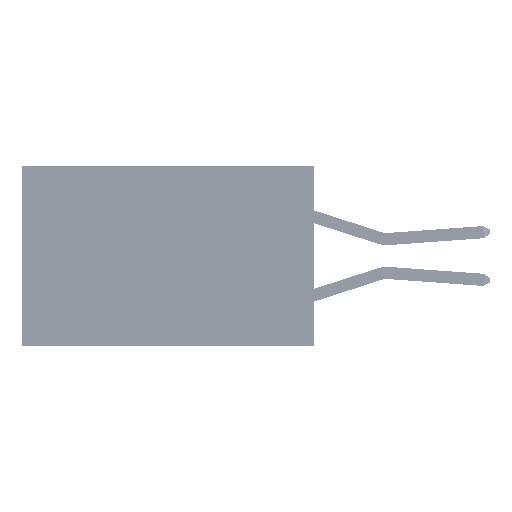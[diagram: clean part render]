
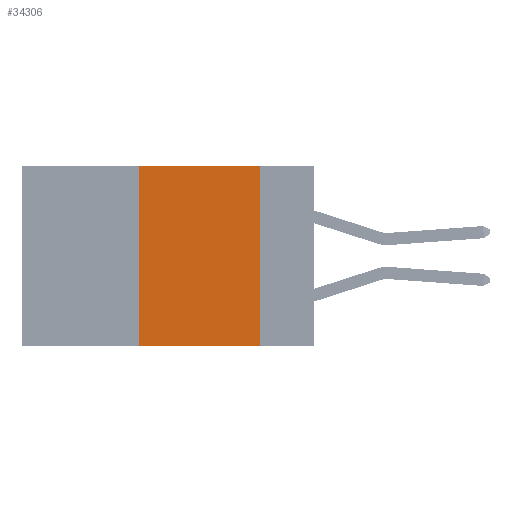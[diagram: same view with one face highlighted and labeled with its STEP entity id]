
A CAD part, left-side view. The second image highlights one B-rep face of the part: STEP entity #34306.
In plain terms, the highlighted planar face has unit normal (-1, 0, 0).
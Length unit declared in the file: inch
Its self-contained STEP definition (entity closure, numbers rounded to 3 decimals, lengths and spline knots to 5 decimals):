
#2879 = FACE_OUTER_BOUND ( 'NONE', #26928, .T. ) ;
#3085 = LINE ( 'NONE', #14199, #21149 ) ;
#3390 = DIRECTION ( 'NONE',  ( 0., 0., -1. ) ) ;
#4465 = AXIS2_PLACEMENT_3D ( 'NONE', #35096, #42013, #3390 ) ;
#5598 = LINE ( 'NONE', #5856, #26160 ) ;
#5856 = CARTESIAN_POINT ( 'NONE',  ( 0., 0.11, 0. ) ) ;
#6752 = ORIENTED_EDGE ( 'NONE', *, *, #8956, .F. ) ;
#7299 = DIRECTION ( 'NONE',  ( 0., 0., 1. ) ) ;
#8205 = CARTESIAN_POINT ( 'NONE',  ( 0., 0.11, 0. ) ) ;
#8956 = EDGE_CURVE ( 'NONE', #11413, #26299, #22181, .T. ) ;
#9167 = ORIENTED_EDGE ( 'NONE', *, *, #14141, .F. ) ;
#9688 = LINE ( 'NONE', #39726, #31656 ) ;
#11413 = VERTEX_POINT ( 'NONE', #16229 ) ;
#13466 = DIRECTION ( 'NONE',  ( 0., -1., 0. ) ) ;
#13785 = VECTOR ( 'NONE', #7299, 39.37008 ) ;
#14141 = EDGE_CURVE ( 'NONE', #20784, #45633, #5598, .T. ) ;
#14199 = CARTESIAN_POINT ( 'NONE',  ( 0., 0.6, 0. ) ) ;
#14696 = DIRECTION ( 'NONE',  ( 0., -1., 0. ) ) ;
#16229 = CARTESIAN_POINT ( 'NONE',  ( 0., 0.36, -0.37 ) ) ;
#17462 = DIRECTION ( 'NONE',  ( 0., 0., -1. ) ) ;
#19686 = PLANE ( 'NONE',  #4465 ) ;
#20784 = VERTEX_POINT ( 'NONE', #8205 ) ;
#21149 = VECTOR ( 'NONE', #14696, 39.37008 ) ;
#22181 = LINE ( 'NONE', #42149, #13785 ) ;
#25736 = ORIENTED_EDGE ( 'NONE', *, *, #46364, .T. ) ;
#26160 = VECTOR ( 'NONE', #17462, 39.37008 ) ;
#26299 = VERTEX_POINT ( 'NONE', #42294 ) ;
#26928 = EDGE_LOOP ( 'NONE', ( #9167, #28516, #6752, #25736 ) ) ;
#28516 = ORIENTED_EDGE ( 'NONE', *, *, #30932, .F. ) ;
#30932 = EDGE_CURVE ( 'NONE', #26299, #20784, #3085, .T. ) ;
#31656 = VECTOR ( 'NONE', #13466, 39.37008 ) ;
#34306 = ADVANCED_FACE ( 'NONE', ( #2879 ), #19686, .F. ) ;
#35096 = CARTESIAN_POINT ( 'NONE',  ( 0., 0.6, 0. ) ) ;
#39726 = CARTESIAN_POINT ( 'NONE',  ( 0., 0.6, -0.37 ) ) ;
#42013 = DIRECTION ( 'NONE',  ( 1., 0., 0. ) ) ;
#42149 = CARTESIAN_POINT ( 'NONE',  ( 0., 0.36, 0. ) ) ;
#42294 = CARTESIAN_POINT ( 'NONE',  ( 0., 0.36, 0. ) ) ;
#45633 = VERTEX_POINT ( 'NONE', #49345 ) ;
#46364 = EDGE_CURVE ( 'NONE', #11413, #45633, #9688, .T. ) ;
#49345 = CARTESIAN_POINT ( 'NONE',  ( 0., 0.11, -0.37 ) ) ;
